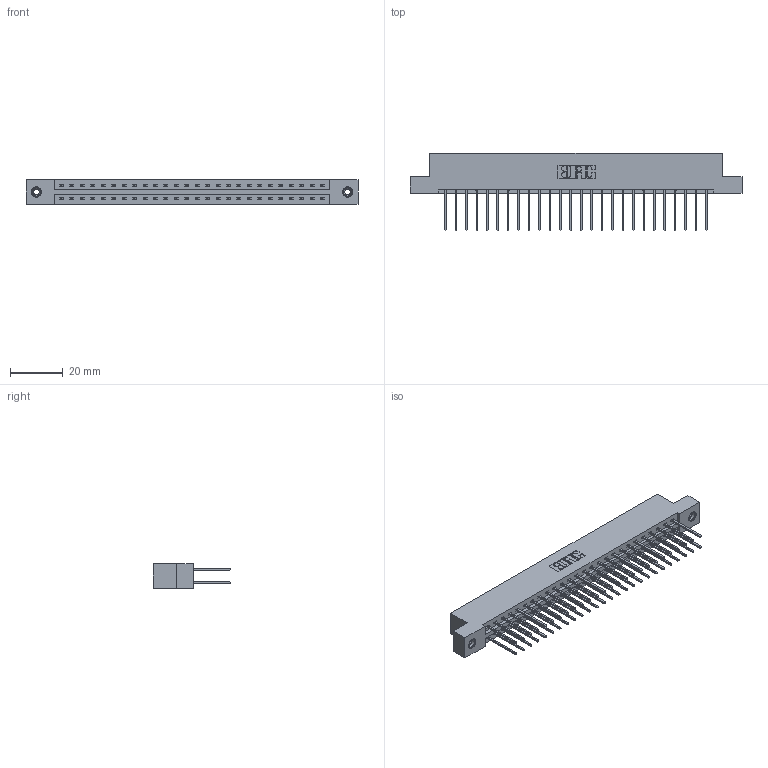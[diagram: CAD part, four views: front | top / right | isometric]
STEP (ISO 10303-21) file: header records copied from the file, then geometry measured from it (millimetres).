
FILE_DESCRIPTION (( 'STEP AP203' ), '1' );
FILE_NAME ('387-052-540-208.STEP', '2019-10-19T03:12:14', ( '' ), ( '' ), 'SwSTEP 2.0', 'SolidWorks 2016', '' );
FILE_SCHEMA (( 'CONFIG_CONTROL_DESIGN' ));
Length unit declared in the file: inch
Products named in the file (4): 345-292-001_345-293-140; 337 Part_Flush Mounting Lugs - 0.156 Dia-TI; 387-052-540-208; 345-250-001_345-250-003-102
Assembly tree (55 placements, depth 2):
  387-052-540-208
    337 Part_Flush Mounting Lugs - 0.156 Dia-TI
    345-292-001_345-293-140  x52
    345-250-001_345-250-003-102  x2
Bounding box: 126.03 x 29.47 x 9.4 mm (x, y, z)
Volume: 13260.2 mm3; surface area: 15833.6 mm2
Topology: 55 solids, 55 shells, 2982 faces, 8819 edges, 5802 vertices
Faces by surface type: plane 2078, cylinder 888, cone 12, torus 4
Entity records: 23432 total; most frequent: CARTESIAN_POINT 3941, ORIENTED_EDGE 3870, DIRECTION 3413, EDGE_CURVE 1935, VECTOR 1787, LINE 1787, VERTEX_POINT 1284, AXIS2_PLACEMENT_3D 813
